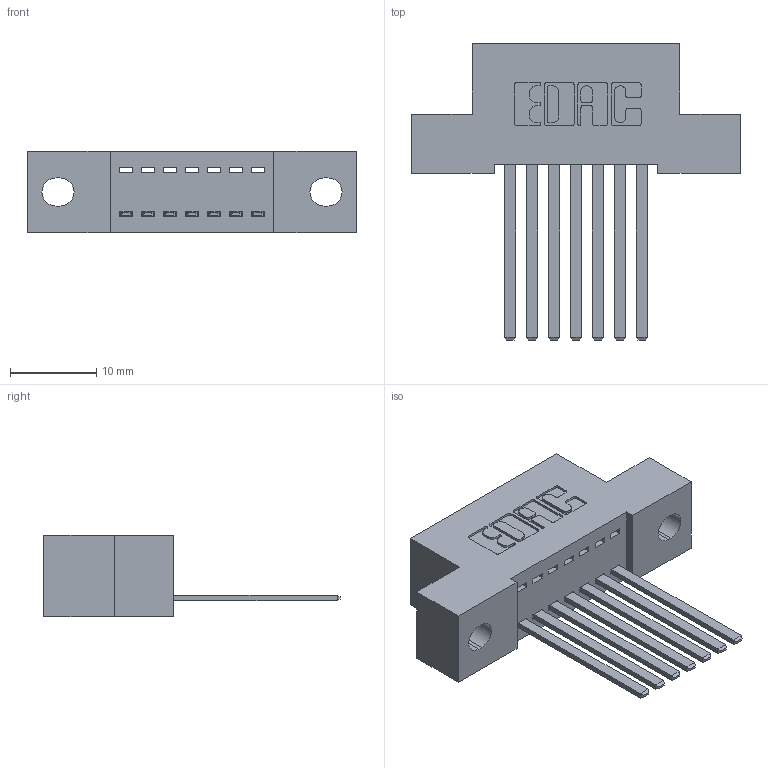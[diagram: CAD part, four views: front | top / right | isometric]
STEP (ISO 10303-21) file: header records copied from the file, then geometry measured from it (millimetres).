
FILE_DESCRIPTION (( 'STEP AP203' ), '1' );
FILE_NAME ('342-007-544-102.STEP', '2019-10-01T12:55:38', ( '' ), ( '' ), 'SwSTEP 2.0', 'SolidWorks 2016', '' );
FILE_SCHEMA (( 'CONFIG_CONTROL_DESIGN' ));
Length unit declared in the file: inch
Products named in the file (3): 342-007-544-102; 342 Part_.128 Slot; 345-292-001_345-293-144
Assembly tree (8 placements, depth 2):
  342-007-544-102
    342 Part_.128 Slot
    345-292-001_345-293-144  x7
Bounding box: 38.1 x 34.3 x 9.4 mm (x, y, z)
Volume: 3240.6 mm3; surface area: 4095.6 mm2
Topology: 8 solids, 8 shells, 478 faces, 1417 edges, 934 vertices
Faces by surface type: plane 336, cylinder 142
Entity records: 8625 total; most frequent: CARTESIAN_POINT 1499, ORIENTED_EDGE 1442, DIRECTION 1331, EDGE_CURVE 721, LINE 597, VECTOR 597, VERTEX_POINT 478, AXIS2_PLACEMENT_3D 367
